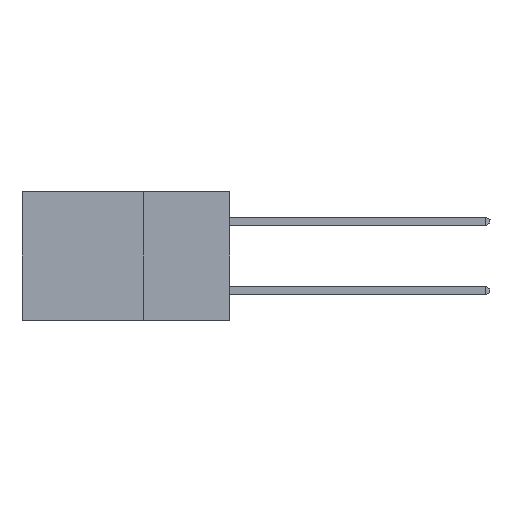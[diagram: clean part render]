
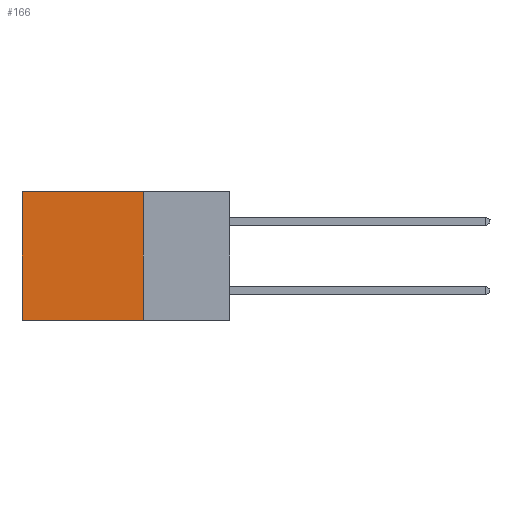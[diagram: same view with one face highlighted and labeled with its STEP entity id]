
A CAD part, left-side view. The second image highlights one B-rep face of the part: STEP entity #166.
In plain terms, the highlighted planar face has unit normal (-1, 0, 0).
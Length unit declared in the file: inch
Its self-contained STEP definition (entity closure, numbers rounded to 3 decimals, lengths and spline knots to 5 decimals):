
#166 = ADVANCED_FACE ( 'NONE', ( #21428 ), #24372, .F. ) ;
#1024 = CARTESIAN_POINT ( 'NONE',  ( 0.298, 0.6, 0. ) ) ;
#1595 = ORIENTED_EDGE ( 'NONE', *, *, #10724, .T. ) ;
#1634 = ORIENTED_EDGE ( 'NONE', *, *, #13576, .T. ) ;
#1962 = VERTEX_POINT ( 'NONE', #5899 ) ;
#2309 = LINE ( 'NONE', #6881, #22176 ) ;
#2439 = CARTESIAN_POINT ( 'NONE',  ( 0.298, 0.25, 0. ) ) ;
#2657 = EDGE_CURVE ( 'NONE', #5786, #6519, #11187, .T. ) ;
#3047 = CARTESIAN_POINT ( 'NONE',  ( 0.298, 0.25, 0. ) ) ;
#3325 = EDGE_LOOP ( 'NONE', ( #1595, #17857, #22132, #1634 ) ) ;
#4982 = DIRECTION ( 'NONE',  ( 1., 0., 0. ) ) ;
#5786 = VERTEX_POINT ( 'NONE', #17880 ) ;
#5899 = CARTESIAN_POINT ( 'NONE',  ( 0.298, 0.6, 0. ) ) ;
#6514 = VECTOR ( 'NONE', #22975, 39.37008 ) ;
#6519 = VERTEX_POINT ( 'NONE', #19808 ) ;
#6702 = DIRECTION ( 'NONE',  ( 0., 0., -1. ) ) ;
#6881 = CARTESIAN_POINT ( 'NONE',  ( 0.298, 0.25, 0. ) ) ;
#6916 = LINE ( 'NONE', #1024, #11184 ) ;
#10724 = EDGE_CURVE ( 'NONE', #1962, #6519, #6916, .T. ) ;
#11184 = VECTOR ( 'NONE', #6702, 39.37008 ) ;
#11187 = LINE ( 'NONE', #20023, #15971 ) ;
#12240 = VERTEX_POINT ( 'NONE', #2439 ) ;
#12809 = EDGE_CURVE ( 'NONE', #12240, #5786, #21010, .T. ) ;
#13576 = EDGE_CURVE ( 'NONE', #12240, #1962, #2309, .T. ) ;
#15971 = VECTOR ( 'NONE', #20518, 39.37008 ) ;
#17157 = AXIS2_PLACEMENT_3D ( 'NONE', #3047, #4982, #18453 ) ;
#17857 = ORIENTED_EDGE ( 'NONE', *, *, #2657, .F. ) ;
#17880 = CARTESIAN_POINT ( 'NONE',  ( 0.298, 0.25, -0.37 ) ) ;
#18453 = DIRECTION ( 'NONE',  ( 0., 0., -1. ) ) ;
#19808 = CARTESIAN_POINT ( 'NONE',  ( 0.298, 0.6, -0.37 ) ) ;
#20023 = CARTESIAN_POINT ( 'NONE',  ( 0.298, 0.25, -0.37 ) ) ;
#20518 = DIRECTION ( 'NONE',  ( 0., 1., 0. ) ) ;
#21010 = LINE ( 'NONE', #21299, #6514 ) ;
#21299 = CARTESIAN_POINT ( 'NONE',  ( 0.298, 0.25, 0. ) ) ;
#21428 = FACE_OUTER_BOUND ( 'NONE', #3325, .T. ) ;
#22132 = ORIENTED_EDGE ( 'NONE', *, *, #12809, .F. ) ;
#22176 = VECTOR ( 'NONE', #24207, 39.37008 ) ;
#22975 = DIRECTION ( 'NONE',  ( 0., 0., -1. ) ) ;
#24207 = DIRECTION ( 'NONE',  ( 0., 1., 0. ) ) ;
#24372 = PLANE ( 'NONE',  #17157 ) ;
